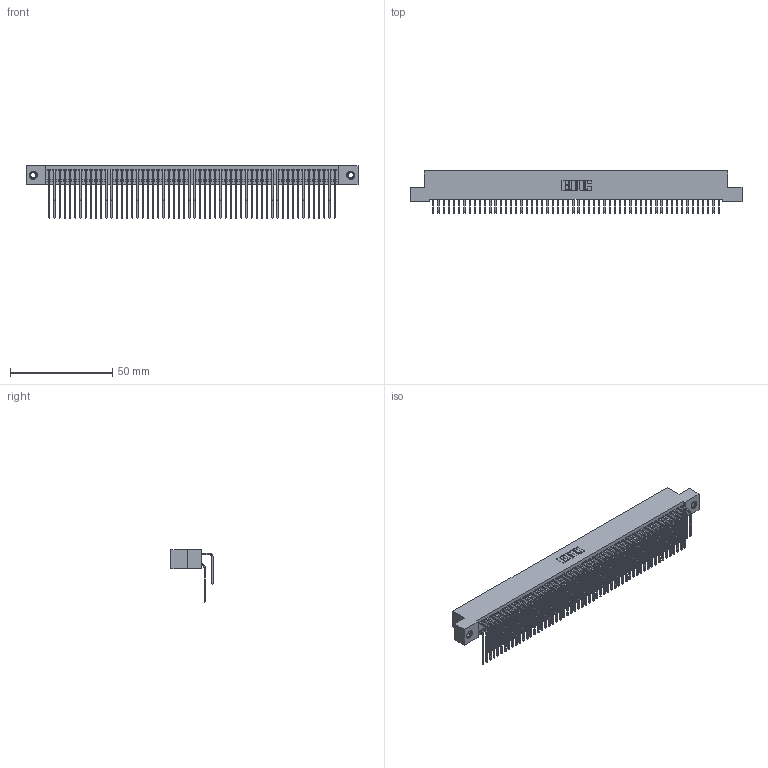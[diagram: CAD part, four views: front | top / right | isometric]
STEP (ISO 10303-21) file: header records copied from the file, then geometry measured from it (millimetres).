
FILE_DESCRIPTION (( 'STEP AP203' ), '1' );
FILE_NAME ('392-112-559-207.STEP', '2019-10-10T00:43:52', ( '' ), ( '' ), 'SwSTEP 2.0', 'SolidWorks 2016', '' );
FILE_SCHEMA (( 'CONFIG_CONTROL_DESIGN' ));
Length unit declared in the file: inch
Products named in the file (5): 392-112-559-207; 342 Part_TI; 345-292-001_558 559 Tail - 1; 345-292-001_559 Tail - 2; 345-250-001_345-250-005-103
Assembly tree (115 placements, depth 2):
  392-112-559-207
    342 Part_TI
    345-292-001_558 559 Tail - 1  x56
    345-292-001_559 Tail - 2  x56
    345-250-001_345-250-005-103  x2
Bounding box: 162.56 x 20.64 x 25.78 mm (x, y, z)
Volume: 15305.7 mm3; surface area: 28207.3 mm2
Topology: 115 solids, 115 shells, 6218 faces, 18467 edges, 12154 vertices
Faces by surface type: plane 4354, cylinder 1848, cone 12, torus 4
Entity records: 37054 total; most frequent: CARTESIAN_POINT 6156, ORIENTED_EDGE 6034, DIRECTION 5247, EDGE_CURVE 3017, LINE 2829, VECTOR 2829, VERTEX_POINT 2004, AXIS2_PLACEMENT_3D 1209
